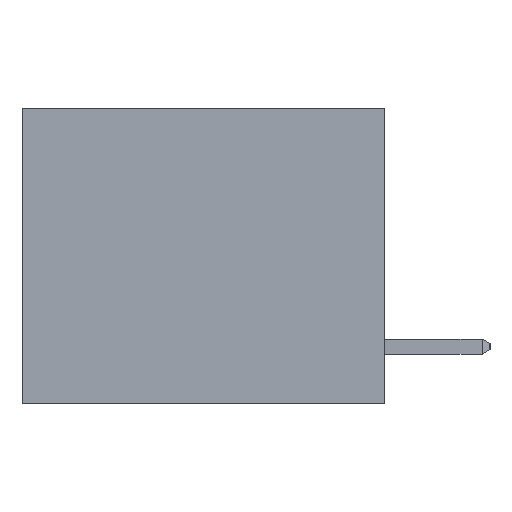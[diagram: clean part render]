
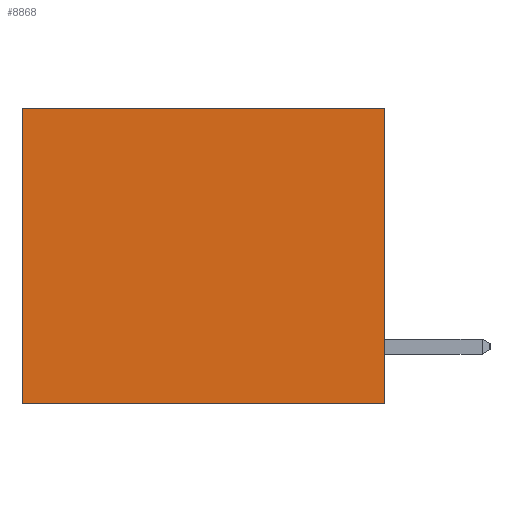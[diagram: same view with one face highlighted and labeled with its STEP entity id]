
A CAD part, left-side view. The second image highlights one B-rep face of the part: STEP entity #8868.
In plain terms, the highlighted planar face has unit normal (-1, 0, 0).
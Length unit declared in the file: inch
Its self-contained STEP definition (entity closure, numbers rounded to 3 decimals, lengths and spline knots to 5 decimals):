
#257 = EDGE_CURVE ( 'NONE', #8777, #12762, #26255, .T. ) ;
#1044 = EDGE_CURVE ( 'NONE', #10680, #23290, #4613, .T. ) ;
#2310 = DIRECTION ( 'NONE',  ( 0., 0., -1. ) ) ;
#3840 = ORIENTED_EDGE ( 'NONE', *, *, #19092, .T. ) ;
#3904 = VECTOR ( 'NONE', #2310, 39.37008 ) ;
#3942 = CARTESIAN_POINT ( 'NONE',  ( 0.3165, 0., 0. ) ) ;
#4613 = LINE ( 'NONE', #3942, #5351 ) ;
#4699 = CARTESIAN_POINT ( 'NONE',  ( 0.3165, 0.6, -0.49 ) ) ;
#4852 = PLANE ( 'NONE',  #12055 ) ;
#4907 = CARTESIAN_POINT ( 'NONE',  ( 0.3165, 0., 0. ) ) ;
#5351 = VECTOR ( 'NONE', #13677, 39.37008 ) ;
#5901 = EDGE_LOOP ( 'NONE', ( #3840, #27651, #29550, #26504 ) ) ;
#6387 = FACE_OUTER_BOUND ( 'NONE', #5901, .T. ) ;
#7241 = CARTESIAN_POINT ( 'NONE',  ( 0.3165, 0., -0.49 ) ) ;
#7990 = CARTESIAN_POINT ( 'NONE',  ( 0.3165, 0., -0.49 ) ) ;
#8777 = VERTEX_POINT ( 'NONE', #20752 ) ;
#8868 = ADVANCED_FACE ( 'NONE', ( #6387 ), #4852, .F. ) ;
#10211 = DIRECTION ( 'NONE',  ( 0., 0., -1. ) ) ;
#10457 = CARTESIAN_POINT ( 'NONE',  ( 0.3165, 0.6, 0. ) ) ;
#10680 = VERTEX_POINT ( 'NONE', #4907 ) ;
#10833 = VECTOR ( 'NONE', #10211, 39.37008 ) ;
#11878 = DIRECTION ( 'NONE',  ( 1., 0., 0. ) ) ;
#12055 = AXIS2_PLACEMENT_3D ( 'NONE', #7241, #11878, #23326 ) ;
#12762 = VERTEX_POINT ( 'NONE', #16728 ) ;
#13310 = EDGE_CURVE ( 'NONE', #10680, #8777, #20166, .T. ) ;
#13677 = DIRECTION ( 'NONE',  ( 0., 1., 0. ) ) ;
#15802 = VECTOR ( 'NONE', #24710, 39.37008 ) ;
#16728 = CARTESIAN_POINT ( 'NONE',  ( 0.3165, 0.6, -0.49 ) ) ;
#17944 = CARTESIAN_POINT ( 'NONE',  ( 0.3165, 0., -0.49 ) ) ;
#19092 = EDGE_CURVE ( 'NONE', #23290, #12762, #21522, .T. ) ;
#20166 = LINE ( 'NONE', #7990, #10833 ) ;
#20752 = CARTESIAN_POINT ( 'NONE',  ( 0.3165, 0., -0.49 ) ) ;
#21522 = LINE ( 'NONE', #4699, #3904 ) ;
#23290 = VERTEX_POINT ( 'NONE', #10457 ) ;
#23326 = DIRECTION ( 'NONE',  ( 0., 0., -1. ) ) ;
#24710 = DIRECTION ( 'NONE',  ( 0., 1., 0. ) ) ;
#26255 = LINE ( 'NONE', #17944, #15802 ) ;
#26504 = ORIENTED_EDGE ( 'NONE', *, *, #1044, .T. ) ;
#27651 = ORIENTED_EDGE ( 'NONE', *, *, #257, .F. ) ;
#29550 = ORIENTED_EDGE ( 'NONE', *, *, #13310, .F. ) ;
